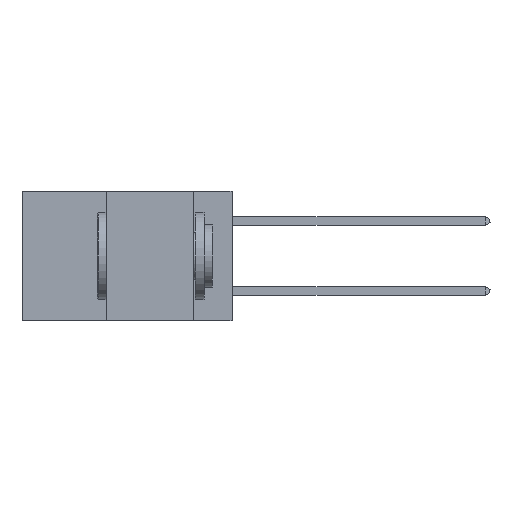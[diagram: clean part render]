
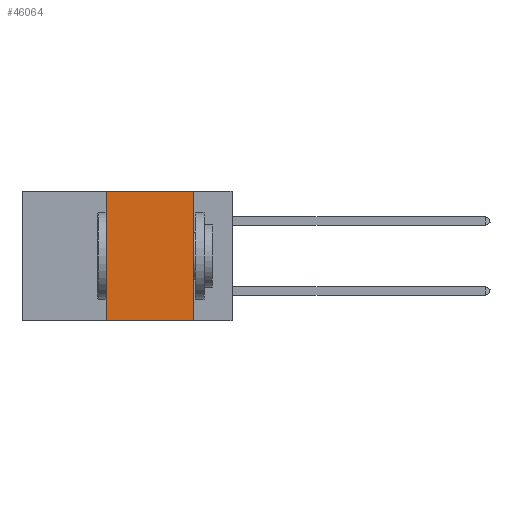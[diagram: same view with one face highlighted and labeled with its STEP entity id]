
A CAD part, left-side view. The second image highlights one B-rep face of the part: STEP entity #46064.
In plain terms, the highlighted planar face has unit normal (-1, 0, 0).
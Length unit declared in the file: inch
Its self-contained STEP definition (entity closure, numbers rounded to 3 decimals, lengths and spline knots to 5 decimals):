
#1252 = VERTEX_POINT ( 'NONE', #28439 ) ;
#1376 = DIRECTION ( 'NONE',  ( 0., 0., 1. ) ) ;
#4614 = EDGE_CURVE ( 'NONE', #42504, #1252, #20804, .T. ) ;
#4862 = DIRECTION ( 'NONE',  ( 1., 0., 0. ) ) ;
#5677 = ORIENTED_EDGE ( 'NONE', *, *, #23391, .F. ) ;
#7093 = VECTOR ( 'NONE', #25355, 39.37008 ) ;
#7436 = DIRECTION ( 'NONE',  ( 0., 0., -1. ) ) ;
#10938 = AXIS2_PLACEMENT_3D ( 'NONE', #22806, #4862, #26968 ) ;
#18071 = VERTEX_POINT ( 'NONE', #45889 ) ;
#18298 = DIRECTION ( 'NONE',  ( 0., -1., 0. ) ) ;
#19260 = EDGE_LOOP ( 'NONE', ( #5677, #37579, #31803, #46151 ) ) ;
#20804 = LINE ( 'NONE', #23364, #37973 ) ;
#22806 = CARTESIAN_POINT ( 'NONE',  ( 0., 0.6, 0. ) ) ;
#23364 = CARTESIAN_POINT ( 'NONE',  ( 0., 0.36, 0. ) ) ;
#23391 = EDGE_CURVE ( 'NONE', #43301, #18071, #32607, .T. ) ;
#25355 = DIRECTION ( 'NONE',  ( 0., -1., 0. ) ) ;
#26016 = CARTESIAN_POINT ( 'NONE',  ( 0., 0.11, 0. ) ) ;
#26813 = PLANE ( 'NONE',  #10938 ) ;
#26877 = EDGE_CURVE ( 'NONE', #42504, #18071, #36855, .T. ) ;
#26968 = DIRECTION ( 'NONE',  ( 0., 0., -1. ) ) ;
#28439 = CARTESIAN_POINT ( 'NONE',  ( 0., 0.36, 0. ) ) ;
#31803 = ORIENTED_EDGE ( 'NONE', *, *, #4614, .F. ) ;
#32059 = CARTESIAN_POINT ( 'NONE',  ( 0., 0.6, 0. ) ) ;
#32477 = FACE_OUTER_BOUND ( 'NONE', #19260, .T. ) ;
#32607 = LINE ( 'NONE', #26016, #42337 ) ;
#33193 = CARTESIAN_POINT ( 'NONE',  ( 0., 0.36, -0.37 ) ) ;
#33761 = CARTESIAN_POINT ( 'NONE',  ( 0., 0.11, 0. ) ) ;
#34018 = LINE ( 'NONE', #32059, #7093 ) ;
#36192 = CARTESIAN_POINT ( 'NONE',  ( 0., 0.6, -0.37 ) ) ;
#36855 = LINE ( 'NONE', #36192, #43148 ) ;
#37579 = ORIENTED_EDGE ( 'NONE', *, *, #42339, .F. ) ;
#37973 = VECTOR ( 'NONE', #1376, 39.37008 ) ;
#42337 = VECTOR ( 'NONE', #7436, 39.37008 ) ;
#42339 = EDGE_CURVE ( 'NONE', #1252, #43301, #34018, .T. ) ;
#42504 = VERTEX_POINT ( 'NONE', #33193 ) ;
#43148 = VECTOR ( 'NONE', #18298, 39.37008 ) ;
#43301 = VERTEX_POINT ( 'NONE', #33761 ) ;
#45889 = CARTESIAN_POINT ( 'NONE',  ( 0., 0.11, -0.37 ) ) ;
#46064 = ADVANCED_FACE ( 'NONE', ( #32477 ), #26813, .F. ) ;
#46151 = ORIENTED_EDGE ( 'NONE', *, *, #26877, .T. ) ;
